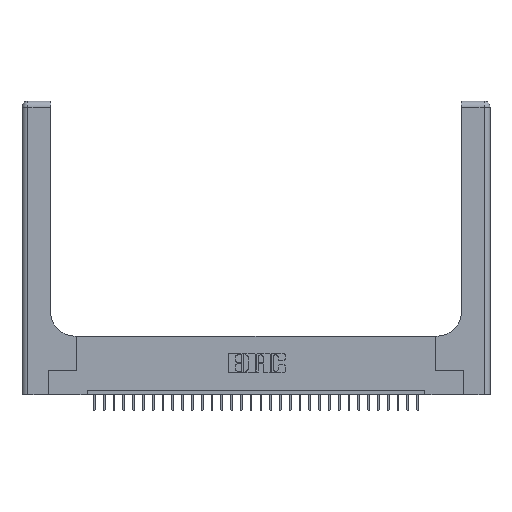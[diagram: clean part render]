
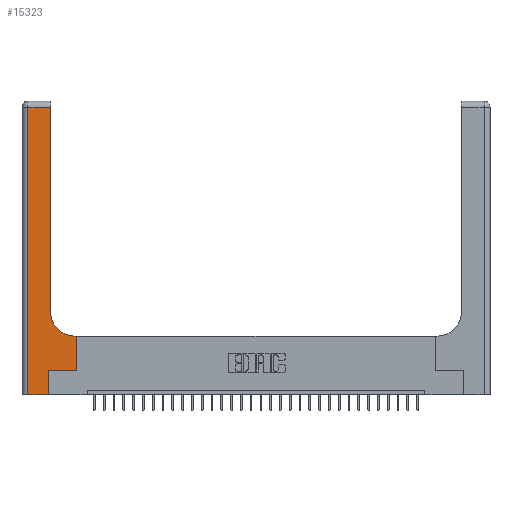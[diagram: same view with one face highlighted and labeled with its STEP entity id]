
A CAD part, top view. The second image highlights one B-rep face of the part: STEP entity #15323.
In plain terms, the highlighted planar face has unit normal (0, 0, 1).
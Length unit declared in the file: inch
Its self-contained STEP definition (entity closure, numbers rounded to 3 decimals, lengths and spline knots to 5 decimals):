
#511 = CARTESIAN_POINT ( 'NONE',  ( 0.2915, 3., 0.37 ) ) ;
#660 = VECTOR ( 'NONE', #20182, 39.37008 ) ;
#815 = ORIENTED_EDGE ( 'NONE', *, *, #22407, .T. ) ;
#1525 = DIRECTION ( 'NONE',  ( -1., 0., 0. ) ) ;
#1732 = ORIENTED_EDGE ( 'NONE', *, *, #30009, .T. ) ;
#2115 = VECTOR ( 'NONE', #3486, 39.37008 ) ;
#3131 = VERTEX_POINT ( 'NONE', #13070 ) ;
#3164 = ORIENTED_EDGE ( 'NONE', *, *, #22008, .T. ) ;
#3182 = VERTEX_POINT ( 'NONE', #19938 ) ;
#3486 = DIRECTION ( 'NONE',  ( 1., 0., 0. ) ) ;
#3638 = CARTESIAN_POINT ( 'NONE',  ( 0., 3., 0.37 ) ) ;
#4351 = LINE ( 'NONE', #30237, #9790 ) ;
#4440 = CARTESIAN_POINT ( 'NONE',  ( 0.5415, 0.6, 0.37 ) ) ;
#4740 = VERTEX_POINT ( 'NONE', #8555 ) ;
#4910 = VECTOR ( 'NONE', #10839, 39.37008 ) ;
#4915 = CARTESIAN_POINT ( 'NONE',  ( 0.2915, 0.6, 0.37 ) ) ;
#5014 = DIRECTION ( 'NONE',  ( -1., 0., 0. ) ) ;
#5679 = LINE ( 'NONE', #6167, #4910 ) ;
#6167 = CARTESIAN_POINT ( 'NONE',  ( 0.5585, 0.25, 0.37 ) ) ;
#6181 = DIRECTION ( 'NONE',  ( 0., 0., -1. ) ) ;
#6696 = ORIENTED_EDGE ( 'NONE', *, *, #8062, .T. ) ;
#7581 = LINE ( 'NONE', #20856, #24578 ) ;
#8008 = EDGE_CURVE ( 'NONE', #18457, #11007, #10992, .T. ) ;
#8062 = EDGE_CURVE ( 'NONE', #11007, #3182, #9039, .T. ) ;
#8555 = CARTESIAN_POINT ( 'NONE',  ( 0.269, 0.25, 0.37 ) ) ;
#9039 = LINE ( 'NONE', #16023, #2115 ) ;
#9317 = EDGE_CURVE ( 'NONE', #3182, #4740, #4351, .T. ) ;
#9651 = ORIENTED_EDGE ( 'NONE', *, *, #11780, .T. ) ;
#9790 = VECTOR ( 'NONE', #24875, 39.37008 ) ;
#9807 = VERTEX_POINT ( 'NONE', #17988 ) ;
#9946 = LINE ( 'NONE', #29583, #31530 ) ;
#10830 = EDGE_CURVE ( 'NONE', #9807, #3131, #5679, .T. ) ;
#10839 = DIRECTION ( 'NONE',  ( 0., 1., 0. ) ) ;
#10992 = LINE ( 'NONE', #13906, #16003 ) ;
#11007 = VERTEX_POINT ( 'NONE', #13468 ) ;
#11110 = DIRECTION ( 'NONE',  ( 0., 0., -1. ) ) ;
#11177 = CIRCLE ( 'NONE', #28374, 0.25 ) ;
#11296 = CARTESIAN_POINT ( 'NONE',  ( 0.5415, 0.85, 0.37 ) ) ;
#11444 = DIRECTION ( 'NONE',  ( 0., -1., 0. ) ) ;
#11780 = EDGE_CURVE ( 'NONE', #26268, #18441, #15665, .T. ) ;
#12111 = CARTESIAN_POINT ( 'NONE',  ( 0.2915, 0.85, 0.37 ) ) ;
#13070 = CARTESIAN_POINT ( 'NONE',  ( 0.5585, 0.6, 0.37 ) ) ;
#13468 = CARTESIAN_POINT ( 'NONE',  ( 0.06, 0., 0.37 ) ) ;
#13906 = CARTESIAN_POINT ( 'NONE',  ( 0.06, 3., 0.37 ) ) ;
#14163 = CARTESIAN_POINT ( 'NONE',  ( 0.06, 2.94, 0.37 ) ) ;
#14837 = DIRECTION ( 'NONE',  ( -1., 0., 0. ) ) ;
#15038 = ORIENTED_EDGE ( 'NONE', *, *, #9317, .T. ) ;
#15323 = ADVANCED_FACE ( 'NONE', ( #20453 ), #16271, .F. ) ;
#15665 = LINE ( 'NONE', #511, #660 ) ;
#15996 = EDGE_CURVE ( 'NONE', #16387, #26268, #11177, .T. ) ;
#16003 = VECTOR ( 'NONE', #11444, 39.37008 ) ;
#16023 = CARTESIAN_POINT ( 'NONE',  ( 0., 0., 0.37 ) ) ;
#16271 = PLANE ( 'NONE',  #24258 ) ;
#16387 = VERTEX_POINT ( 'NONE', #4440 ) ;
#17988 = CARTESIAN_POINT ( 'NONE',  ( 0.5585, 0.25, 0.37 ) ) ;
#18441 = VERTEX_POINT ( 'NONE', #18731 ) ;
#18457 = VERTEX_POINT ( 'NONE', #14163 ) ;
#18731 = CARTESIAN_POINT ( 'NONE',  ( 0.2915, 2.94, 0.37 ) ) ;
#19938 = CARTESIAN_POINT ( 'NONE',  ( 0.269, 0., 0.37 ) ) ;
#20182 = DIRECTION ( 'NONE',  ( 0., 1., 0. ) ) ;
#20453 = FACE_OUTER_BOUND ( 'NONE', #29798, .T. ) ;
#20856 = CARTESIAN_POINT ( 'NONE',  ( 0.269, 0.25, 0.37 ) ) ;
#22008 = EDGE_CURVE ( 'NONE', #3131, #16387, #29973, .T. ) ;
#22407 = EDGE_CURVE ( 'NONE', #18441, #18457, #9946, .T. ) ;
#23571 = DIRECTION ( 'NONE',  ( 1., 0., 0. ) ) ;
#24258 = AXIS2_PLACEMENT_3D ( 'NONE', #3638, #11110, #1525 ) ;
#24578 = VECTOR ( 'NONE', #23571, 39.37008 ) ;
#24875 = DIRECTION ( 'NONE',  ( 0., 1., 0. ) ) ;
#24930 = ORIENTED_EDGE ( 'NONE', *, *, #8008, .T. ) ;
#25933 = ORIENTED_EDGE ( 'NONE', *, *, #15996, .T. ) ;
#26268 = VERTEX_POINT ( 'NONE', #12111 ) ;
#28255 = DIRECTION ( 'NONE',  ( 1., 0., 0. ) ) ;
#28374 = AXIS2_PLACEMENT_3D ( 'NONE', #11296, #6181, #28255 ) ;
#29583 = CARTESIAN_POINT ( 'NONE',  ( 0., 2.94, 0.37 ) ) ;
#29636 = ORIENTED_EDGE ( 'NONE', *, *, #10830, .T. ) ;
#29798 = EDGE_LOOP ( 'NONE', ( #9651, #815, #24930, #6696, #15038, #1732, #29636, #3164, #25933 ) ) ;
#29973 = LINE ( 'NONE', #4915, #30768 ) ;
#30009 = EDGE_CURVE ( 'NONE', #4740, #9807, #7581, .T. ) ;
#30237 = CARTESIAN_POINT ( 'NONE',  ( 0.269, 0., 0.37 ) ) ;
#30768 = VECTOR ( 'NONE', #5014, 39.37008 ) ;
#31530 = VECTOR ( 'NONE', #14837, 39.37008 ) ;
